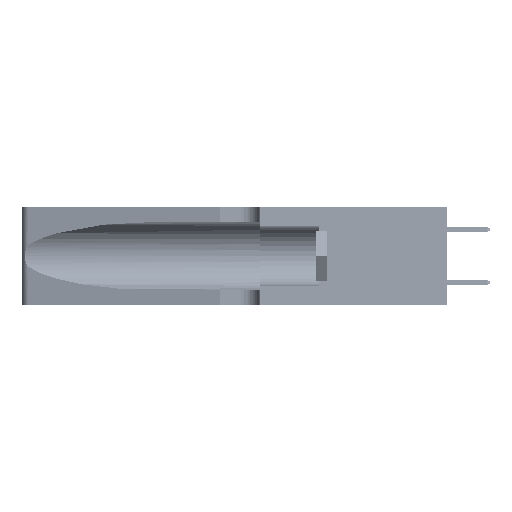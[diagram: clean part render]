
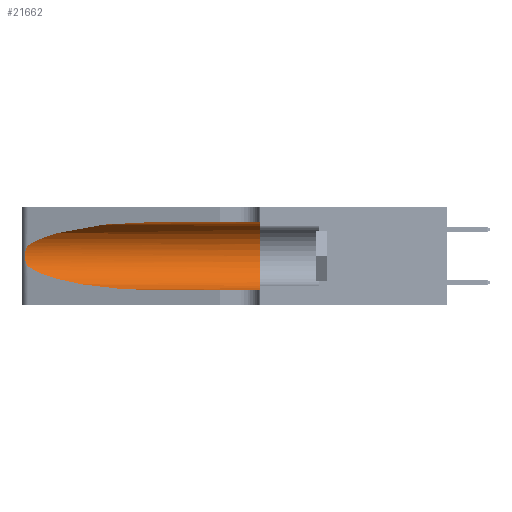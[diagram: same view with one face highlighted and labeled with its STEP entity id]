
A CAD part, left-side view. The second image highlights one B-rep face of the part: STEP entity #21662.
In plain terms, the highlighted cylindrical face has radius 3.308 mm (diameter 6.617 mm), a partial arc.
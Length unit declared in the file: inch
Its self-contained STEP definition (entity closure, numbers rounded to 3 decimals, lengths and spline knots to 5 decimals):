
#1376 = VERTEX_POINT ( 'NONE', #12827 ) ;
#1932 = CARTESIAN_POINT ( 'NONE',  ( 0.1305, 0.72297, 0.31525 ) ) ;
#2262 = DIRECTION ( 'NONE',  ( 0., 0., 1. ) ) ;
#4424 = CARTESIAN_POINT ( 'NONE',  ( 0.25787, 1.23484, 0.2124 ) ) ;
#4453 =( BOUNDED_CURVE ( )  B_SPLINE_CURVE ( 3, ( #35308, #47363, #19038, #47545 ),
 .UNSPECIFIED., .F., .F. ) 
 B_SPLINE_CURVE_WITH_KNOTS ( ( 4, 4 ),
 ( 3.44316, 4.71239 ),
 .UNSPECIFIED. ) 
 CURVE ( )  GEOMETRIC_REPRESENTATION_ITEM ( )  RATIONAL_B_SPLINE_CURVE ( ( 1., 0.87, 0.87, 1. ) ) 
 REPRESENTATION_ITEM ( '' )  );
#5201 = CYLINDRICAL_SURFACE ( 'NONE', #50002, 0.13025 ) ;
#5522 = CARTESIAN_POINT ( 'NONE',  ( 0.1305, 1.61858, 0.185 ) ) ;
#6476 = AXIS2_PLACEMENT_3D ( 'NONE', #51193, #26812, #2262 ) ;
#7285 = ORIENTED_EDGE ( 'NONE', *, *, #13860, .F. ) ;
#7337 = VERTEX_POINT ( 'NONE', #23345 ) ;
#8455 = VERTEX_POINT ( 'NONE', #13929 ) ;
#8546 = CARTESIAN_POINT ( 'NONE',  ( 0.26018, 1.23835, 0.19895 ) ) ;
#9283 = DIRECTION ( 'NONE',  ( 0., -1., 0. ) ) ;
#9592 = LINE ( 'NONE', #21978, #19218 ) ;
#10194 = CARTESIAN_POINT ( 'NONE',  ( 0.2373, 1.15595, 0.28018 ) ) ;
#11913 = ORIENTED_EDGE ( 'NONE', *, *, #32641, .T. ) ;
#12656 = CARTESIAN_POINT ( 'NONE',  ( 0.26075, 1.23896, 0.178 ) ) ;
#12827 = CARTESIAN_POINT ( 'NONE',  ( 0.1305, 0.35, 0.05475 ) ) ;
#13027 = ORIENTED_EDGE ( 'NONE', *, *, #29519, .F. ) ;
#13629 = CIRCLE ( 'NONE', #6476, 0.13025 ) ;
#13860 = EDGE_CURVE ( 'NONE', #21267, #14267, #9592, .T. ) ;
#13894 = VERTEX_POINT ( 'NONE', #14105 ) ;
#13929 = CARTESIAN_POINT ( 'NONE',  ( 0.25487, 1.22718, 0.14631 ) ) ;
#13989 =( BOUNDED_CURVE ( )  B_SPLINE_CURVE ( 3, ( #1932, #26480, #10194, #38780 ),
 .UNSPECIFIED., .F., .F. ) 
 B_SPLINE_CURVE_WITH_KNOTS ( ( 4, 4 ),
 ( 1.5708, 2.84003 ),
 .UNSPECIFIED. ) 
 CURVE ( )  GEOMETRIC_REPRESENTATION_ITEM ( )  RATIONAL_B_SPLINE_CURVE ( ( 1., 0.87, 0.87, 1. ) ) 
 REPRESENTATION_ITEM ( '' )  );
#14105 = CARTESIAN_POINT ( 'NONE',  ( 0.1305, 0.72297, 0.05475 ) ) ;
#14267 = VERTEX_POINT ( 'NONE', #16534 ) ;
#16534 = CARTESIAN_POINT ( 'NONE',  ( 0.1305, 0.35, 0.31525 ) ) ;
#16766 = CARTESIAN_POINT ( 'NONE',  ( 0.25856, 1.23593, 0.16098 ) ) ;
#17691 = CARTESIAN_POINT ( 'NONE',  ( 0.1305, 1.61858, 0.05475 ) ) ;
#19038 = CARTESIAN_POINT ( 'NONE',  ( 0.18966, 0.96281, 0.05475 ) ) ;
#19218 = VECTOR ( 'NONE', #38221, 39.37008 ) ;
#20729 = CARTESIAN_POINT ( 'NONE',  ( 0.25487, 1.22718, 0.22369 ) ) ;
#20910 = CARTESIAN_POINT ( 'NONE',  ( 0.25639, 1.23186, 0.15144 ) ) ;
#21267 = VERTEX_POINT ( 'NONE', #27426 ) ;
#21662 = ADVANCED_FACE ( 'NONE', ( #26992 ), #5201, .F. ) ;
#21978 = CARTESIAN_POINT ( 'NONE',  ( 0.1305, 1.61858, 0.31525 ) ) ;
#22585 = VECTOR ( 'NONE', #38234, 39.37008 ) ;
#23345 = CARTESIAN_POINT ( 'NONE',  ( 0.25487, 1.22718, 0.22369 ) ) ;
#24906 = EDGE_CURVE ( 'NONE', #7337, #8455, #49106, .T. ) ;
#25014 = CARTESIAN_POINT ( 'NONE',  ( 0.25487, 1.22718, 0.14631 ) ) ;
#25169 = ORIENTED_EDGE ( 'NONE', *, *, #42682, .T. ) ;
#26480 = CARTESIAN_POINT ( 'NONE',  ( 0.18966, 0.96281, 0.31525 ) ) ;
#26812 = DIRECTION ( 'NONE',  ( 0., 1., 0. ) ) ;
#26992 = FACE_OUTER_BOUND ( 'NONE', #50279, .T. ) ;
#27426 = CARTESIAN_POINT ( 'NONE',  ( 0.1305, 0.72297, 0.31525 ) ) ;
#28953 = CARTESIAN_POINT ( 'NONE',  ( 0.25639, 1.23184, 0.21858 ) ) ;
#29519 = EDGE_CURVE ( 'NONE', #14267, #1376, #13629, .T. ) ;
#32344 = ORIENTED_EDGE ( 'NONE', *, *, #24906, .T. ) ;
#32641 = EDGE_CURVE ( 'NONE', #13894, #1376, #39178, .T. ) ;
#33055 = CARTESIAN_POINT ( 'NONE',  ( 0.25854, 1.2359, 0.20912 ) ) ;
#35308 = CARTESIAN_POINT ( 'NONE',  ( 0.25487, 1.22718, 0.14631 ) ) ;
#35309 = EDGE_CURVE ( 'NONE', #21267, #7337, #13989, .T. ) ;
#37165 = CARTESIAN_POINT ( 'NONE',  ( 0.26075, 1.23896, 0.19203 ) ) ;
#37896 = DIRECTION ( 'NONE',  ( 0., 0., -1. ) ) ;
#38221 = DIRECTION ( 'NONE',  ( 0., -1., 0. ) ) ;
#38234 = DIRECTION ( 'NONE',  ( 0., -1., 0. ) ) ;
#38780 = CARTESIAN_POINT ( 'NONE',  ( 0.25487, 1.22718, 0.22369 ) ) ;
#39178 = LINE ( 'NONE', #17691, #22585 ) ;
#41218 = CARTESIAN_POINT ( 'NONE',  ( 0.26017, 1.23833, 0.17102 ) ) ;
#42682 = EDGE_CURVE ( 'NONE', #8455, #13894, #4453, .T. ) ;
#45122 = CARTESIAN_POINT ( 'NONE',  ( 0.25555, 1.22994, 0.2215 ) ) ;
#45292 = CARTESIAN_POINT ( 'NONE',  ( 0.25789, 1.23486, 0.15765 ) ) ;
#47363 = CARTESIAN_POINT ( 'NONE',  ( 0.2373, 1.15595, 0.08982 ) ) ;
#47545 = CARTESIAN_POINT ( 'NONE',  ( 0.1305, 0.72297, 0.05475 ) ) ;
#49106 = B_SPLINE_CURVE_WITH_KNOTS ( 'NONE', 3,
 ( #20729, #45122, #28953, #4424, #33055, #8546, #37165, #12656, #41218, #16766, #45292, #20910, #49399, #25014 ),
 .UNSPECIFIED., .F., .F.,
 ( 4, 2, 2, 2, 2, 2, 4 ),
 ( 0., 0.00027, 0.00053, 0.00107, 0.0016, 0.00187, 0.00214 ),
 .UNSPECIFIED. ) ;
#49399 = CARTESIAN_POINT ( 'NONE',  ( 0.25555, 1.22993, 0.14849 ) ) ;
#50002 = AXIS2_PLACEMENT_3D ( 'NONE', #5522, #9283, #37896 ) ;
#50279 = EDGE_LOOP ( 'NONE', ( #52792, #32344, #25169, #11913, #13027, #7285 ) ) ;
#51193 = CARTESIAN_POINT ( 'NONE',  ( 0.1305, 0.35, 0.185 ) ) ;
#52792 = ORIENTED_EDGE ( 'NONE', *, *, #35309, .T. ) ;
